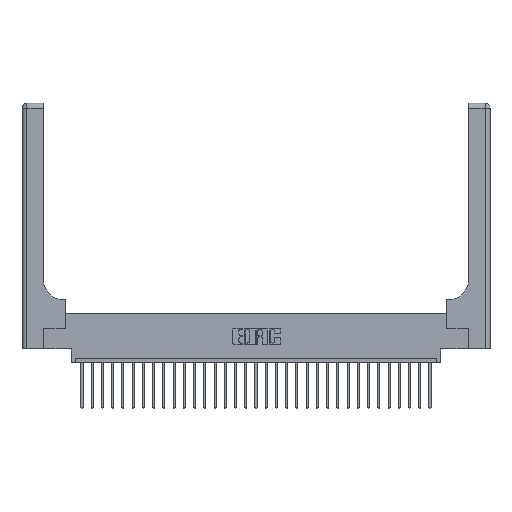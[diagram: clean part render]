
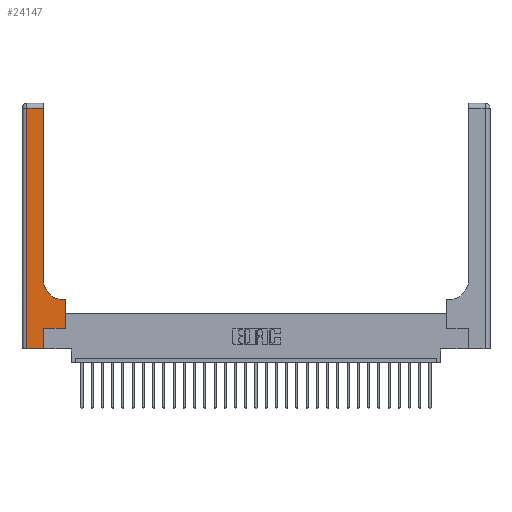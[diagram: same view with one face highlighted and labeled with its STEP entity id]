
A CAD part, top view. The second image highlights one B-rep face of the part: STEP entity #24147.
In plain terms, the highlighted planar face has unit normal (0, 0, 1).
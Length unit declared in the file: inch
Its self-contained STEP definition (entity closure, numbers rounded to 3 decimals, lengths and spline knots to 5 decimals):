
#1286 = VERTEX_POINT ( 'NONE', #19729 ) ;
#1590 = ORIENTED_EDGE ( 'NONE', *, *, #8614, .T. ) ;
#1751 = EDGE_CURVE ( 'NONE', #24890, #24043, #4854, .T. ) ;
#2013 = CARTESIAN_POINT ( 'NONE',  ( 0.265, 0.25, 0.37 ) ) ;
#2146 = FACE_OUTER_BOUND ( 'NONE', #3829, .T. ) ;
#2708 = ORIENTED_EDGE ( 'NONE', *, *, #22831, .T. ) ;
#3180 = DIRECTION ( 'NONE',  ( 0., 0., -1. ) ) ;
#3429 = CARTESIAN_POINT ( 'NONE',  ( 0.06, 0., 0.37 ) ) ;
#3467 = VECTOR ( 'NONE', #24677, 39.37008 ) ;
#3729 = ORIENTED_EDGE ( 'NONE', *, *, #20986, .T. ) ;
#3829 = EDGE_LOOP ( 'NONE', ( #19210, #18088, #1590, #26419, #22375, #2708, #17582, #3729, #9586 ) ) ;
#4854 = LINE ( 'NONE', #11740, #9598 ) ;
#5051 = EDGE_CURVE ( 'NONE', #28023, #8675, #12451, .T. ) ;
#6348 = CARTESIAN_POINT ( 'NONE',  ( 0.06, 3., 0.37 ) ) ;
#6808 = VECTOR ( 'NONE', #25853, 39.37008 ) ;
#7446 = CARTESIAN_POINT ( 'NONE',  ( 0.528, 0.25, 0.37 ) ) ;
#7632 = CARTESIAN_POINT ( 'NONE',  ( 0.528, 0.6, 0.37 ) ) ;
#8614 = EDGE_CURVE ( 'NONE', #19135, #24890, #17934, .T. ) ;
#8675 = VERTEX_POINT ( 'NONE', #17646 ) ;
#9195 = LINE ( 'NONE', #7446, #3467 ) ;
#9586 = ORIENTED_EDGE ( 'NONE', *, *, #5051, .T. ) ;
#9598 = VECTOR ( 'NONE', #15764, 39.37008 ) ;
#9601 = EDGE_CURVE ( 'NONE', #8675, #23049, #16187, .T. ) ;
#9917 = LINE ( 'NONE', #27134, #24717 ) ;
#10220 = VECTOR ( 'NONE', #11887, 39.37008 ) ;
#11131 = DIRECTION ( 'NONE',  ( -1., 0., 0. ) ) ;
#11740 = CARTESIAN_POINT ( 'NONE',  ( 0., 0., 0.37 ) ) ;
#11844 = CARTESIAN_POINT ( 'NONE',  ( 0.26, 0.6, 0.37 ) ) ;
#11887 = DIRECTION ( 'NONE',  ( 0., 1., 0. ) ) ;
#12451 = CIRCLE ( 'NONE', #21359, 0.25 ) ;
#13324 = CARTESIAN_POINT ( 'NONE',  ( 0.528, 0.25, 0.37 ) ) ;
#13411 = VERTEX_POINT ( 'NONE', #7632 ) ;
#14818 = DIRECTION ( 'NONE',  ( 1., 0., 0. ) ) ;
#14895 = LINE ( 'NONE', #22609, #10220 ) ;
#15248 = PLANE ( 'NONE',  #18311 ) ;
#15764 = DIRECTION ( 'NONE',  ( 1., 0., 0. ) ) ;
#15904 = CARTESIAN_POINT ( 'NONE',  ( 0.06, 2.94, 0.37 ) ) ;
#16121 = LINE ( 'NONE', #11844, #23587 ) ;
#16187 = LINE ( 'NONE', #25046, #18232 ) ;
#16539 = VERTEX_POINT ( 'NONE', #13324 ) ;
#17149 = CARTESIAN_POINT ( 'NONE',  ( 0.265, 0., 0.37 ) ) ;
#17413 = EDGE_CURVE ( 'NONE', #16539, #13411, #9195, .T. ) ;
#17441 = EDGE_CURVE ( 'NONE', #24043, #1286, #14895, .T. ) ;
#17582 = ORIENTED_EDGE ( 'NONE', *, *, #17413, .T. ) ;
#17646 = CARTESIAN_POINT ( 'NONE',  ( 0.26, 0.85, 0.37 ) ) ;
#17934 = LINE ( 'NONE', #6348, #6808 ) ;
#18088 = ORIENTED_EDGE ( 'NONE', *, *, #24289, .T. ) ;
#18232 = VECTOR ( 'NONE', #18524, 39.37008 ) ;
#18306 = DIRECTION ( 'NONE',  ( -1., 0., 0. ) ) ;
#18311 = AXIS2_PLACEMENT_3D ( 'NONE', #23923, #21754, #11131 ) ;
#18524 = DIRECTION ( 'NONE',  ( 0., 1., 0. ) ) ;
#19135 = VERTEX_POINT ( 'NONE', #15904 ) ;
#19210 = ORIENTED_EDGE ( 'NONE', *, *, #9601, .T. ) ;
#19729 = CARTESIAN_POINT ( 'NONE',  ( 0.265, 0.25, 0.37 ) ) ;
#20986 = EDGE_CURVE ( 'NONE', #13411, #28023, #16121, .T. ) ;
#21359 = AXIS2_PLACEMENT_3D ( 'NONE', #27073, #3180, #22963 ) ;
#21754 = DIRECTION ( 'NONE',  ( 0., 0., -1. ) ) ;
#22375 = ORIENTED_EDGE ( 'NONE', *, *, #17441, .T. ) ;
#22609 = CARTESIAN_POINT ( 'NONE',  ( 0.265, 0., 0.37 ) ) ;
#22831 = EDGE_CURVE ( 'NONE', #1286, #16539, #26513, .T. ) ;
#22963 = DIRECTION ( 'NONE',  ( 1., 0., 0. ) ) ;
#23049 = VERTEX_POINT ( 'NONE', #26808 ) ;
#23587 = VECTOR ( 'NONE', #27132, 39.37008 ) ;
#23923 = CARTESIAN_POINT ( 'NONE',  ( 0., 3., 0.37 ) ) ;
#24043 = VERTEX_POINT ( 'NONE', #17149 ) ;
#24147 = ADVANCED_FACE ( 'NONE', ( #2146 ), #15248, .F. ) ;
#24289 = EDGE_CURVE ( 'NONE', #23049, #19135, #9917, .T. ) ;
#24677 = DIRECTION ( 'NONE',  ( 0., 1., 0. ) ) ;
#24717 = VECTOR ( 'NONE', #18306, 39.37008 ) ;
#24890 = VERTEX_POINT ( 'NONE', #3429 ) ;
#25046 = CARTESIAN_POINT ( 'NONE',  ( 0.26, 3., 0.37 ) ) ;
#25220 = CARTESIAN_POINT ( 'NONE',  ( 0.51, 0.6, 0.37 ) ) ;
#25853 = DIRECTION ( 'NONE',  ( 0., -1., 0. ) ) ;
#26179 = VECTOR ( 'NONE', #14818, 39.37008 ) ;
#26419 = ORIENTED_EDGE ( 'NONE', *, *, #1751, .T. ) ;
#26513 = LINE ( 'NONE', #2013, #26179 ) ;
#26808 = CARTESIAN_POINT ( 'NONE',  ( 0.26, 2.94, 0.37 ) ) ;
#27073 = CARTESIAN_POINT ( 'NONE',  ( 0.51, 0.85, 0.37 ) ) ;
#27132 = DIRECTION ( 'NONE',  ( -1., 0., 0. ) ) ;
#27134 = CARTESIAN_POINT ( 'NONE',  ( 0., 2.94, 0.37 ) ) ;
#28023 = VERTEX_POINT ( 'NONE', #25220 ) ;
